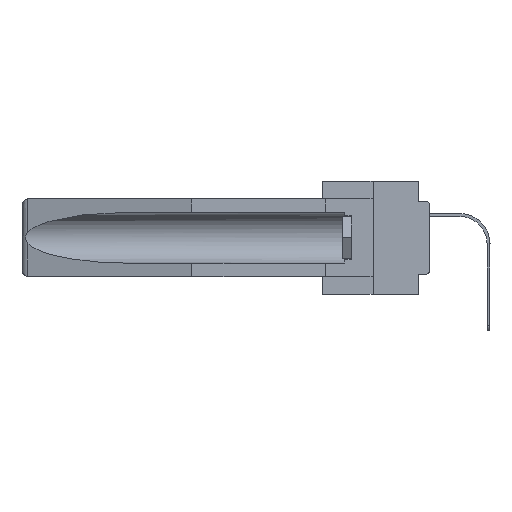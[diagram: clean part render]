
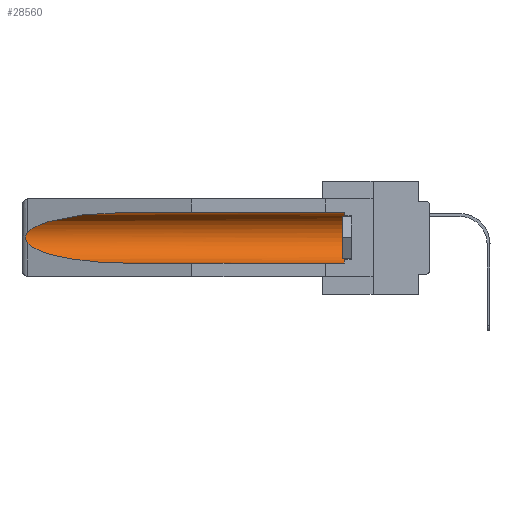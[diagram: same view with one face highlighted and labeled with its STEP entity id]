
A CAD part, left-side view. The second image highlights one B-rep face of the part: STEP entity #28560.
In plain terms, the highlighted cylindrical face has radius 2.857 mm (diameter 5.715 mm), a partial arc.
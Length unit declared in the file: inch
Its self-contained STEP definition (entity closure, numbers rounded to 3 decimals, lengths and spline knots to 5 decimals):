
#1179 = CIRCLE ( 'NONE', #17967, 0.1125 ) ;
#1571 = DIRECTION ( 'NONE',  ( 0., -1., 0. ) ) ;
#1712 = CARTESIAN_POINT ( 'NONE',  ( 0.2673, 1.5327, -0.16383 ) ) ;
#1859 = CARTESIAN_POINT ( 'NONE',  ( 0.26655, 1.53094, -0.18657 ) ) ;
#2751 = B_SPLINE_CURVE_WITH_KNOTS ( 'NONE', 3,
 ( #24437, #3280, #27354, #1712, #3871, #18403, #25497, #1859, #25351, #23024 ),
 .UNSPECIFIED., .F., .F.,
 ( 4, 2, 2, 2, 4 ),
 ( 0., 0.00029, 0.00058, 0.00087, 0.00117 ),
 .UNSPECIFIED. ) ;
#2943 = CARTESIAN_POINT ( 'NONE',  ( 0.25451, 1.48313, -0.09465 ) ) ;
#3243 = CARTESIAN_POINT ( 'NONE',  ( 0.26537, 1.52718, -0.19328 ) ) ;
#3280 = CARTESIAN_POINT ( 'NONE',  ( 0.26597, 1.52961, -0.15275 ) ) ;
#3871 = CARTESIAN_POINT ( 'NONE',  ( 0.2675, 1.53308, -0.16763 ) ) ;
#3936 = EDGE_CURVE ( 'NONE', #27069, #25249, #2751, .T. ) ;
#5192 = EDGE_CURVE ( 'NONE', #10758, #26634, #1179, .T. ) ;
#7742 = ORIENTED_EDGE ( 'NONE', *, *, #5192, .T. ) ;
#8361 = CARTESIAN_POINT ( 'NONE',  ( 0.21114, 1.30732, -0.284 ) ) ;
#8625 = CARTESIAN_POINT ( 'NONE',  ( 0.155, -0.30754, -0.059 ) ) ;
#9232 = ORIENTED_EDGE ( 'NONE', *, *, #26115, .F. ) ;
#10381 = CARTESIAN_POINT ( 'NONE',  ( 0.155, -0.30754, -0.1715 ) ) ;
#10758 = VERTEX_POINT ( 'NONE', #11034 ) ;
#11034 = CARTESIAN_POINT ( 'NONE',  ( 0.155, 0.126, -0.284 ) ) ;
#11125 = CARTESIAN_POINT ( 'NONE',  ( 0.26537, 1.52718, -0.19328 ) ) ;
#11439 =( BOUNDED_CURVE ( )  B_SPLINE_CURVE ( 3, ( #11125, #15764, #8361, #15920 ),
 .UNSPECIFIED., .F., .T. ) 
 B_SPLINE_CURVE_WITH_KNOTS ( ( 4, 4 ),
 ( 0.1948, 1.5708 ),
 .UNSPECIFIED. ) 
 CURVE ( )  GEOMETRIC_REPRESENTATION_ITEM ( )  RATIONAL_B_SPLINE_CURVE ( ( 1., 0.848, 0.848, 1. ) ) 
 REPRESENTATION_ITEM ( '' )  );
#11485 = CARTESIAN_POINT ( 'NONE',  ( 0.155, 1.07973, -0.059 ) ) ;
#11623 = CARTESIAN_POINT ( 'NONE',  ( 0.26537, 1.52718, -0.14972 ) ) ;
#12792 = VERTEX_POINT ( 'NONE', #27271 ) ;
#15052 = DIRECTION ( 'NONE',  ( 0., 1., 0. ) ) ;
#15764 = CARTESIAN_POINT ( 'NONE',  ( 0.25451, 1.48313, -0.24835 ) ) ;
#15920 = CARTESIAN_POINT ( 'NONE',  ( 0.155, 1.07973, -0.284 ) ) ;
#16228 = CARTESIAN_POINT ( 'NONE',  ( 0.155, 0.126, -0.1715 ) ) ;
#17566 = CARTESIAN_POINT ( 'NONE',  ( 0.26537, 1.52718, -0.14972 ) ) ;
#17942 = DIRECTION ( 'NONE',  ( 0., 0., 1. ) ) ;
#17967 = AXIS2_PLACEMENT_3D ( 'NONE', #16228, #1571, #30116 ) ;
#17971 = VECTOR ( 'NONE', #15052, 39.37008 ) ;
#18403 = CARTESIAN_POINT ( 'NONE',  ( 0.2675, 1.53308, -0.17534 ) ) ;
#19331 = CARTESIAN_POINT ( 'NONE',  ( 0.21114, 1.30732, -0.059 ) ) ;
#19631 = CARTESIAN_POINT ( 'NONE',  ( 0.155, 0.126, -0.059 ) ) ;
#19702 = LINE ( 'NONE', #26349, #17971 ) ;
#19856 = VECTOR ( 'NONE', #25310, 39.37008 ) ;
#21009 = VERTEX_POINT ( 'NONE', #24402 ) ;
#22031 = AXIS2_PLACEMENT_3D ( 'NONE', #10381, #29647, #17942 ) ;
#22571 = CYLINDRICAL_SURFACE ( 'NONE', #22031, 0.1125 ) ;
#23024 = CARTESIAN_POINT ( 'NONE',  ( 0.26537, 1.52718, -0.19328 ) ) ;
#23705 = EDGE_CURVE ( 'NONE', #25249, #12792, #11439, .T. ) ;
#24113 = EDGE_CURVE ( 'NONE', #26634, #21009, #27771, .T. ) ;
#24402 = CARTESIAN_POINT ( 'NONE',  ( 0.155, 1.07973, -0.059 ) ) ;
#24433 = FACE_OUTER_BOUND ( 'NONE', #27478, .T. ) ;
#24437 = CARTESIAN_POINT ( 'NONE',  ( 0.26537, 1.52718, -0.14972 ) ) ;
#24520 = ORIENTED_EDGE ( 'NONE', *, *, #3936, .T. ) ;
#25249 = VERTEX_POINT ( 'NONE', #3243 ) ;
#25310 = DIRECTION ( 'NONE',  ( 0., 1., 0. ) ) ;
#25351 = CARTESIAN_POINT ( 'NONE',  ( 0.26597, 1.5296, -0.19026 ) ) ;
#25497 = CARTESIAN_POINT ( 'NONE',  ( 0.2673, 1.53269, -0.17917 ) ) ;
#25869 = ORIENTED_EDGE ( 'NONE', *, *, #26352, .T. ) ;
#26115 = EDGE_CURVE ( 'NONE', #10758, #12792, #19702, .T. ) ;
#26349 = CARTESIAN_POINT ( 'NONE',  ( 0.155, -0.30754, -0.284 ) ) ;
#26352 = EDGE_CURVE ( 'NONE', #21009, #27069, #27404, .T. ) ;
#26502 = ORIENTED_EDGE ( 'NONE', *, *, #23705, .T. ) ;
#26634 = VERTEX_POINT ( 'NONE', #19631 ) ;
#27069 = VERTEX_POINT ( 'NONE', #17566 ) ;
#27271 = CARTESIAN_POINT ( 'NONE',  ( 0.155, 1.07973, -0.284 ) ) ;
#27354 = CARTESIAN_POINT ( 'NONE',  ( 0.26654, 1.53092, -0.15636 ) ) ;
#27404 =( BOUNDED_CURVE ( )  B_SPLINE_CURVE ( 3, ( #11485, #19331, #2943, #11623 ),
 .UNSPECIFIED., .F., .T. ) 
 B_SPLINE_CURVE_WITH_KNOTS ( ( 4, 4 ),
 ( 4.71239, 6.08839 ),
 .UNSPECIFIED. ) 
 CURVE ( )  GEOMETRIC_REPRESENTATION_ITEM ( )  RATIONAL_B_SPLINE_CURVE ( ( 1., 0.848, 0.848, 1. ) ) 
 REPRESENTATION_ITEM ( '' )  );
#27478 = EDGE_LOOP ( 'NONE', ( #25869, #24520, #26502, #9232, #7742, #29923 ) ) ;
#27771 = LINE ( 'NONE', #8625, #19856 ) ;
#28560 = ADVANCED_FACE ( 'NONE', ( #24433 ), #22571, .F. ) ;
#29647 = DIRECTION ( 'NONE',  ( 0., 1., 0. ) ) ;
#29923 = ORIENTED_EDGE ( 'NONE', *, *, #24113, .T. ) ;
#30116 = DIRECTION ( 'NONE',  ( 0., 0., 1. ) ) ;
